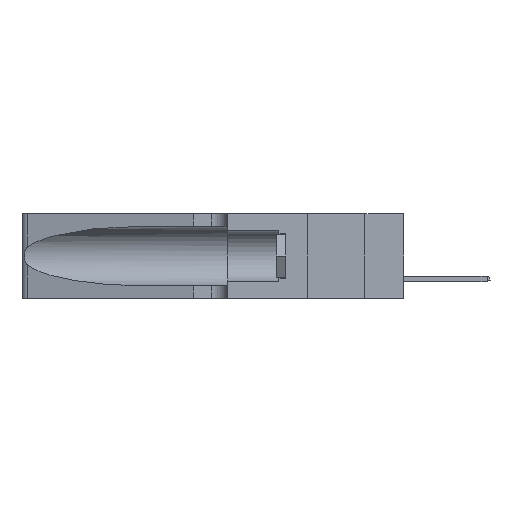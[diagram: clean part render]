
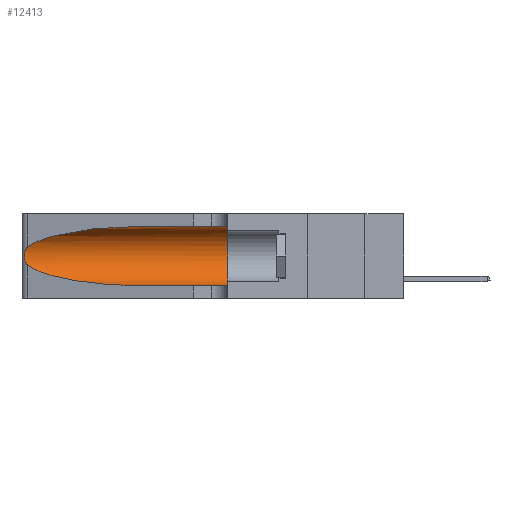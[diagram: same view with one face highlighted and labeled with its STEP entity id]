
A CAD part, left-side view. The second image highlights one B-rep face of the part: STEP entity #12413.
In plain terms, the highlighted cylindrical face has radius 3.308 mm (diameter 6.617 mm), a partial arc.
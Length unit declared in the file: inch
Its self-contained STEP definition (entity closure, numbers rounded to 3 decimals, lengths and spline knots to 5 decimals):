
#324 = CARTESIAN_POINT ( 'NONE',  ( 0.25856, 1.23593, 0.16098 ) ) ;
#570 = CARTESIAN_POINT ( 'NONE',  ( 0.26075, 1.23896, 0.178 ) ) ;
#685 = CARTESIAN_POINT ( 'NONE',  ( 0.25787, 1.23484, 0.2124 ) ) ;
#1420 = VERTEX_POINT ( 'NONE', #32187 ) ;
#1919 = CARTESIAN_POINT ( 'NONE',  ( 0.25487, 1.22718, 0.22369 ) ) ;
#2567 = CARTESIAN_POINT ( 'NONE',  ( 0.25487, 1.22718, 0.22369 ) ) ;
#2880 = CARTESIAN_POINT ( 'NONE',  ( 0.26017, 1.23833, 0.17102 ) ) ;
#4476 =( BOUNDED_CURVE ( )  B_SPLINE_CURVE ( 3, ( #13459, #28560, #20820, #26140 ),
 .UNSPECIFIED., .F., .F. ) 
 B_SPLINE_CURVE_WITH_KNOTS ( ( 4, 4 ),
 ( 3.44316, 4.71239 ),
 .UNSPECIFIED. ) 
 CURVE ( )  GEOMETRIC_REPRESENTATION_ITEM ( )  RATIONAL_B_SPLINE_CURVE ( ( 1., 0.87, 0.87, 1. ) ) 
 REPRESENTATION_ITEM ( '' )  );
#5126 = ORIENTED_EDGE ( 'NONE', *, *, #30989, .T. ) ;
#5823 = CARTESIAN_POINT ( 'NONE',  ( 0.25639, 1.23186, 0.15144 ) ) ;
#5958 = FACE_OUTER_BOUND ( 'NONE', #28578, .T. ) ;
#6436 = ORIENTED_EDGE ( 'NONE', *, *, #13182, .F. ) ;
#6768 = CARTESIAN_POINT ( 'NONE',  ( 0.1305, 0.72297, 0.31525 ) ) ;
#7649 = EDGE_CURVE ( 'NONE', #8072, #1420, #10971, .T. ) ;
#8072 = VERTEX_POINT ( 'NONE', #25396 ) ;
#8189 = CARTESIAN_POINT ( 'NONE',  ( 0.25854, 1.2359, 0.20912 ) ) ;
#8297 = CARTESIAN_POINT ( 'NONE',  ( 0.25639, 1.23184, 0.21858 ) ) ;
#9577 = DIRECTION ( 'NONE',  ( 0., -1., 0. ) ) ;
#10049 = CARTESIAN_POINT ( 'NONE',  ( 0.1305, 1.61858, 0.185 ) ) ;
#10068 = CARTESIAN_POINT ( 'NONE',  ( 0.1305, 0.35, 0.05475 ) ) ;
#10581 = AXIS2_PLACEMENT_3D ( 'NONE', #19441, #14820, #11974 ) ;
#10857 = CARTESIAN_POINT ( 'NONE',  ( 0.26075, 1.23896, 0.19203 ) ) ;
#10971 = B_SPLINE_CURVE_WITH_KNOTS ( 'NONE', 3,
 ( #2567, #22555, #8297, #685, #8189, #28164, #10857, #570, #2880, #324, #13056, #5823, #23542, #28615 ),
 .UNSPECIFIED., .F., .F.,
 ( 4, 2, 2, 2, 2, 2, 4 ),
 ( 0., 0.00027, 0.00053, 0.00107, 0.0016, 0.00187, 0.00214 ),
 .UNSPECIFIED. ) ;
#11974 = DIRECTION ( 'NONE',  ( 0., 0., 1. ) ) ;
#12413 = ADVANCED_FACE ( 'NONE', ( #5958 ), #16261, .F. ) ;
#12652 = EDGE_CURVE ( 'NONE', #27859, #8072, #18222, .T. ) ;
#12732 = VERTEX_POINT ( 'NONE', #10068 ) ;
#13056 = CARTESIAN_POINT ( 'NONE',  ( 0.25789, 1.23486, 0.15765 ) ) ;
#13182 = EDGE_CURVE ( 'NONE', #27859, #19962, #30030, .T. ) ;
#13459 = CARTESIAN_POINT ( 'NONE',  ( 0.25487, 1.22718, 0.14631 ) ) ;
#13503 = ORIENTED_EDGE ( 'NONE', *, *, #28889, .F. ) ;
#14518 = CARTESIAN_POINT ( 'NONE',  ( 0.2373, 1.15595, 0.28018 ) ) ;
#14820 = DIRECTION ( 'NONE',  ( 0., 1., 0. ) ) ;
#15088 = DIRECTION ( 'NONE',  ( 0., -1., 0. ) ) ;
#15114 = DIRECTION ( 'NONE',  ( 0., 0., -1. ) ) ;
#16261 = CYLINDRICAL_SURFACE ( 'NONE', #26918, 0.13025 ) ;
#17112 = CARTESIAN_POINT ( 'NONE',  ( 0.1305, 0.72297, 0.31525 ) ) ;
#17452 = CIRCLE ( 'NONE', #10581, 0.13025 ) ;
#18222 =( BOUNDED_CURVE ( )  B_SPLINE_CURVE ( 3, ( #6768, #27414, #14518, #1919 ),
 .UNSPECIFIED., .F., .T. ) 
 B_SPLINE_CURVE_WITH_KNOTS ( ( 4, 4 ),
 ( 1.5708, 2.84003 ),
 .UNSPECIFIED. ) 
 CURVE ( )  GEOMETRIC_REPRESENTATION_ITEM ( )  RATIONAL_B_SPLINE_CURVE ( ( 1., 0.87, 0.87, 1. ) ) 
 REPRESENTATION_ITEM ( '' )  );
#19441 = CARTESIAN_POINT ( 'NONE',  ( 0.1305, 0.35, 0.185 ) ) ;
#19962 = VERTEX_POINT ( 'NONE', #27425 ) ;
#19964 = DIRECTION ( 'NONE',  ( 0., -1., 0. ) ) ;
#20820 = CARTESIAN_POINT ( 'NONE',  ( 0.18966, 0.96281, 0.05475 ) ) ;
#22267 = CARTESIAN_POINT ( 'NONE',  ( 0.1305, 1.61858, 0.31525 ) ) ;
#22278 = ORIENTED_EDGE ( 'NONE', *, *, #7649, .T. ) ;
#22555 = CARTESIAN_POINT ( 'NONE',  ( 0.25555, 1.22994, 0.2215 ) ) ;
#22806 = CARTESIAN_POINT ( 'NONE',  ( 0.1305, 0.72297, 0.05475 ) ) ;
#22813 = VECTOR ( 'NONE', #9577, 39.37008 ) ;
#23292 = EDGE_CURVE ( 'NONE', #31822, #12732, #30832, .T. ) ;
#23542 = CARTESIAN_POINT ( 'NONE',  ( 0.25555, 1.22993, 0.14849 ) ) ;
#23559 = ORIENTED_EDGE ( 'NONE', *, *, #12652, .T. ) ;
#23724 = VECTOR ( 'NONE', #15088, 39.37008 ) ;
#24695 = CARTESIAN_POINT ( 'NONE',  ( 0.1305, 1.61858, 0.05475 ) ) ;
#25396 = CARTESIAN_POINT ( 'NONE',  ( 0.25487, 1.22718, 0.22369 ) ) ;
#26140 = CARTESIAN_POINT ( 'NONE',  ( 0.1305, 0.72297, 0.05475 ) ) ;
#26250 = ORIENTED_EDGE ( 'NONE', *, *, #23292, .T. ) ;
#26918 = AXIS2_PLACEMENT_3D ( 'NONE', #10049, #19964, #15114 ) ;
#27414 = CARTESIAN_POINT ( 'NONE',  ( 0.18966, 0.96281, 0.31525 ) ) ;
#27425 = CARTESIAN_POINT ( 'NONE',  ( 0.1305, 0.35, 0.31525 ) ) ;
#27859 = VERTEX_POINT ( 'NONE', #17112 ) ;
#28164 = CARTESIAN_POINT ( 'NONE',  ( 0.26018, 1.23835, 0.19895 ) ) ;
#28560 = CARTESIAN_POINT ( 'NONE',  ( 0.2373, 1.15595, 0.08982 ) ) ;
#28578 = EDGE_LOOP ( 'NONE', ( #23559, #22278, #5126, #26250, #13503, #6436 ) ) ;
#28615 = CARTESIAN_POINT ( 'NONE',  ( 0.25487, 1.22718, 0.14631 ) ) ;
#28889 = EDGE_CURVE ( 'NONE', #19962, #12732, #17452, .T. ) ;
#30030 = LINE ( 'NONE', #22267, #23724 ) ;
#30832 = LINE ( 'NONE', #24695, #22813 ) ;
#30989 = EDGE_CURVE ( 'NONE', #1420, #31822, #4476, .T. ) ;
#31822 = VERTEX_POINT ( 'NONE', #22806 ) ;
#32187 = CARTESIAN_POINT ( 'NONE',  ( 0.25487, 1.22718, 0.14631 ) ) ;
